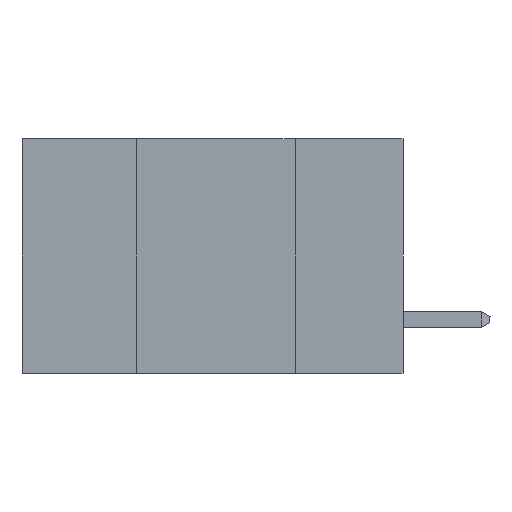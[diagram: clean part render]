
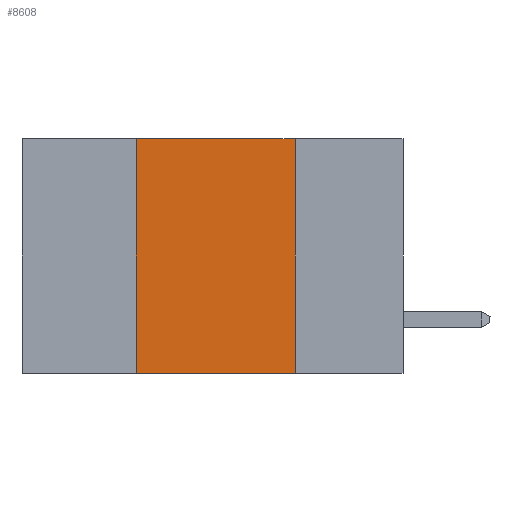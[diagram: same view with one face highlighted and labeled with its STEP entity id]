
A CAD part, left-side view. The second image highlights one B-rep face of the part: STEP entity #8608.
In plain terms, the highlighted planar face has unit normal (-1, 0, 0).
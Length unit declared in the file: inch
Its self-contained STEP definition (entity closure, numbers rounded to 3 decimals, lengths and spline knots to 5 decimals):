
#241 = CARTESIAN_POINT ( 'NONE',  ( 0., 0.6, 0. ) ) ;
#426 = CARTESIAN_POINT ( 'NONE',  ( 0., 0.6, 0. ) ) ;
#429 = VERTEX_POINT ( 'NONE', #5041 ) ;
#1328 = ORIENTED_EDGE ( 'NONE', *, *, #20935, .F. ) ;
#3506 = LINE ( 'NONE', #9179, #13388 ) ;
#3555 = ORIENTED_EDGE ( 'NONE', *, *, #24414, .F. ) ;
#5041 = CARTESIAN_POINT ( 'NONE',  ( 0., 0.17, -0.37 ) ) ;
#6448 = LINE ( 'NONE', #426, #11801 ) ;
#7112 = VECTOR ( 'NONE', #11459, 39.37008 ) ;
#7216 = CARTESIAN_POINT ( 'NONE',  ( 0., 0.42, 0. ) ) ;
#7308 = EDGE_CURVE ( 'NONE', #17921, #429, #22925, .T. ) ;
#7530 = EDGE_CURVE ( 'NONE', #21832, #14992, #6448, .T. ) ;
#7585 = DIRECTION ( 'NONE',  ( 0., 0., -1. ) ) ;
#7714 = FACE_OUTER_BOUND ( 'NONE', #22198, .T. ) ;
#8267 = DIRECTION ( 'NONE',  ( 0., -1., 0. ) ) ;
#8608 = ADVANCED_FACE ( 'NONE', ( #7714 ), #12077, .F. ) ;
#9179 = CARTESIAN_POINT ( 'NONE',  ( 0., 0.17, 0. ) ) ;
#10014 = DIRECTION ( 'NONE',  ( 1., 0., 0. ) ) ;
#11459 = DIRECTION ( 'NONE',  ( 0., 0., 1. ) ) ;
#11801 = VECTOR ( 'NONE', #8267, 39.37008 ) ;
#12077 = PLANE ( 'NONE',  #14281 ) ;
#12592 = CARTESIAN_POINT ( 'NONE',  ( 0., 0.42, -0.37 ) ) ;
#13388 = VECTOR ( 'NONE', #19045, 39.37008 ) ;
#14281 = AXIS2_PLACEMENT_3D ( 'NONE', #241, #10014, #7585 ) ;
#14418 = CARTESIAN_POINT ( 'NONE',  ( 0., 0.17, 0. ) ) ;
#14973 = CARTESIAN_POINT ( 'NONE',  ( 0., 0.42, 0. ) ) ;
#14992 = VERTEX_POINT ( 'NONE', #14418 ) ;
#17921 = VERTEX_POINT ( 'NONE', #12592 ) ;
#18901 = LINE ( 'NONE', #7216, #7112 ) ;
#19045 = DIRECTION ( 'NONE',  ( 0., 0., -1. ) ) ;
#19420 = ORIENTED_EDGE ( 'NONE', *, *, #7530, .F. ) ;
#19831 = ORIENTED_EDGE ( 'NONE', *, *, #7308, .T. ) ;
#20935 = EDGE_CURVE ( 'NONE', #17921, #21832, #18901, .T. ) ;
#21832 = VERTEX_POINT ( 'NONE', #14973 ) ;
#22069 = VECTOR ( 'NONE', #22675, 39.37008 ) ;
#22198 = EDGE_LOOP ( 'NONE', ( #3555, #19420, #1328, #19831 ) ) ;
#22675 = DIRECTION ( 'NONE',  ( 0., -1., 0. ) ) ;
#22925 = LINE ( 'NONE', #24726, #22069 ) ;
#24414 = EDGE_CURVE ( 'NONE', #14992, #429, #3506, .T. ) ;
#24726 = CARTESIAN_POINT ( 'NONE',  ( 0., 0.6, -0.37 ) ) ;
